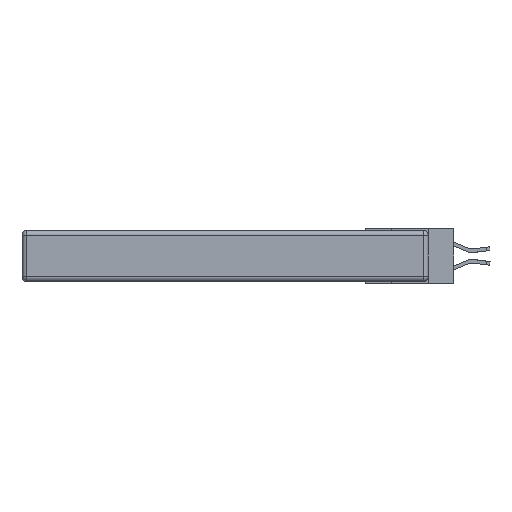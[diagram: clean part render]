
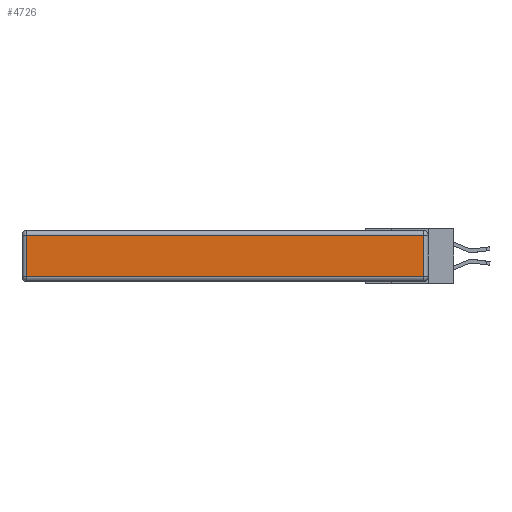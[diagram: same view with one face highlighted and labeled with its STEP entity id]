
A CAD part, left-side view. The second image highlights one B-rep face of the part: STEP entity #4726.
In plain terms, the highlighted planar face has unit normal (-1, 0, 0).
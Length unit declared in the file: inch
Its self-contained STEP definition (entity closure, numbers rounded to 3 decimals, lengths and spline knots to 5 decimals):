
#535 = DIRECTION ( 'NONE',  ( 0., 1., 0. ) ) ;
#900 = ORIENTED_EDGE ( 'NONE', *, *, #4852, .T. ) ;
#1155 = DIRECTION ( 'NONE',  ( -1., 0., 0. ) ) ;
#1276 = FACE_OUTER_BOUND ( 'NONE', #11590, .T. ) ;
#1588 = ORIENTED_EDGE ( 'NONE', *, *, #7299, .T. ) ;
#2399 = VECTOR ( 'NONE', #535, 39.37008 ) ;
#2645 = LINE ( 'NONE', #3835, #7071 ) ;
#2768 = DIRECTION ( 'NONE',  ( 0., -1., 0. ) ) ;
#3298 = EDGE_CURVE ( 'NONE', #6077, #7458, #11932, .T. ) ;
#3381 = DIRECTION ( 'NONE',  ( 0., 0., 1. ) ) ;
#3437 = DIRECTION ( 'NONE',  ( 0., 0., 1. ) ) ;
#3835 = CARTESIAN_POINT ( 'NONE',  ( 0., 0., -0.313 ) ) ;
#4726 = ADVANCED_FACE ( 'NONE', ( #1276 ), #7868, .T. ) ;
#4852 = EDGE_CURVE ( 'NONE', #12969, #6077, #11895, .T. ) ;
#5415 = CARTESIAN_POINT ( 'NONE',  ( 0., 2.75, -0.03 ) ) ;
#5607 = DIRECTION ( 'NONE',  ( 0., 0., -1. ) ) ;
#5808 = ORIENTED_EDGE ( 'NONE', *, *, #9166, .T. ) ;
#6077 = VERTEX_POINT ( 'NONE', #8622 ) ;
#6655 = VECTOR ( 'NONE', #3437, 39.37008 ) ;
#7071 = VECTOR ( 'NONE', #2768, 39.37008 ) ;
#7299 = EDGE_CURVE ( 'NONE', #8380, #12969, #2645, .T. ) ;
#7458 = VERTEX_POINT ( 'NONE', #12128 ) ;
#7501 = CARTESIAN_POINT ( 'NONE',  ( 0., 2.72, -0.343 ) ) ;
#7718 = ORIENTED_EDGE ( 'NONE', *, *, #3298, .T. ) ;
#7769 = AXIS2_PLACEMENT_3D ( 'NONE', #10932, #1155, #3381 ) ;
#7868 = PLANE ( 'NONE',  #7769 ) ;
#8047 = LINE ( 'NONE', #7501, #12523 ) ;
#8380 = VERTEX_POINT ( 'NONE', #13064 ) ;
#8622 = CARTESIAN_POINT ( 'NONE',  ( 0., 0.03, -0.03 ) ) ;
#9166 = EDGE_CURVE ( 'NONE', #7458, #8380, #8047, .T. ) ;
#10268 = CARTESIAN_POINT ( 'NONE',  ( 0., 0.03, -0.313 ) ) ;
#10932 = CARTESIAN_POINT ( 'NONE',  ( 0., 0., -0.343 ) ) ;
#11590 = EDGE_LOOP ( 'NONE', ( #1588, #900, #7718, #5808 ) ) ;
#11684 = CARTESIAN_POINT ( 'NONE',  ( 0., 0.03, -0.343 ) ) ;
#11895 = LINE ( 'NONE', #11684, #6655 ) ;
#11932 = LINE ( 'NONE', #5415, #2399 ) ;
#12128 = CARTESIAN_POINT ( 'NONE',  ( 0., 2.72, -0.03 ) ) ;
#12523 = VECTOR ( 'NONE', #5607, 39.37008 ) ;
#12969 = VERTEX_POINT ( 'NONE', #10268 ) ;
#13064 = CARTESIAN_POINT ( 'NONE',  ( 0., 2.72, -0.313 ) ) ;
